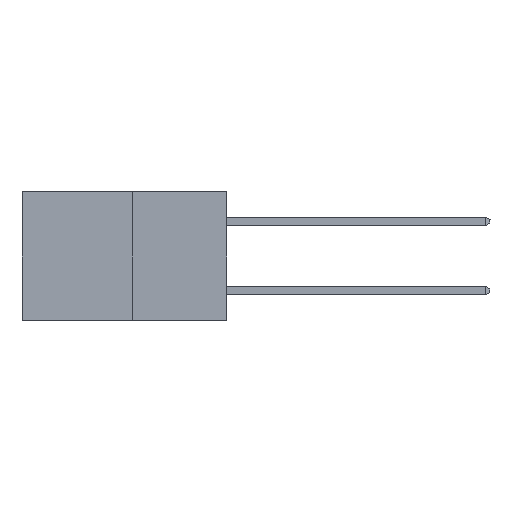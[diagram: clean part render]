
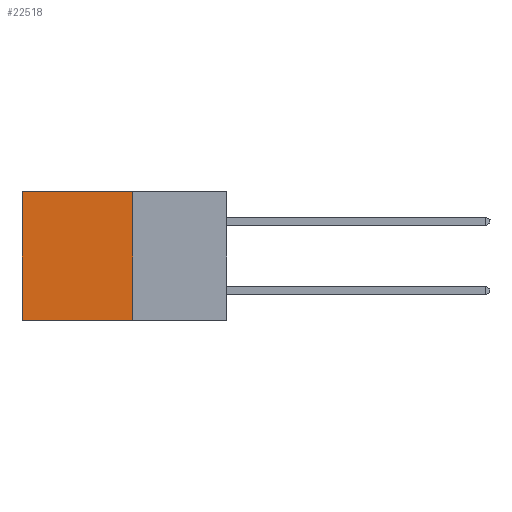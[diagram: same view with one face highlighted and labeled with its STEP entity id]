
A CAD part, left-side view. The second image highlights one B-rep face of the part: STEP entity #22518.
In plain terms, the highlighted planar face has unit normal (-1, 0, 0).
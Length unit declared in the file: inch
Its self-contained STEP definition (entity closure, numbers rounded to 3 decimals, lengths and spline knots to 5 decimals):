
#194 = DIRECTION ( 'NONE',  ( 0., 1., 0. ) ) ;
#245 = CARTESIAN_POINT ( 'NONE',  ( 0.277, 0.27, -0.37 ) ) ;
#1360 = LINE ( 'NONE', #20377, #14068 ) ;
#1440 = VERTEX_POINT ( 'NONE', #5201 ) ;
#2664 = DIRECTION ( 'NONE',  ( 0., 0., -1. ) ) ;
#4241 = ORIENTED_EDGE ( 'NONE', *, *, #16851, .F. ) ;
#5201 = CARTESIAN_POINT ( 'NONE',  ( 0.277, 0.27, 0. ) ) ;
#6169 = VECTOR ( 'NONE', #10595, 39.37008 ) ;
#6457 = EDGE_LOOP ( 'NONE', ( #22980, #4241, #10217, #19124 ) ) ;
#6992 = LINE ( 'NONE', #8060, #6169 ) ;
#8060 = CARTESIAN_POINT ( 'NONE',  ( 0.277, 0.27, 0. ) ) ;
#8202 = VERTEX_POINT ( 'NONE', #9850 ) ;
#9850 = CARTESIAN_POINT ( 'NONE',  ( 0.277, 0.27, -0.37 ) ) ;
#10217 = ORIENTED_EDGE ( 'NONE', *, *, #29340, .F. ) ;
#10595 = DIRECTION ( 'NONE',  ( 0., 1., 0. ) ) ;
#11838 = DIRECTION ( 'NONE',  ( 1., 0., 0. ) ) ;
#14068 = VECTOR ( 'NONE', #2664, 39.37008 ) ;
#14224 = VECTOR ( 'NONE', #194, 39.37008 ) ;
#14652 = LINE ( 'NONE', #245, #27182 ) ;
#15370 = CARTESIAN_POINT ( 'NONE',  ( 0.277, 0.27, -0.37 ) ) ;
#16851 = EDGE_CURVE ( 'NONE', #8202, #30140, #20117, .T. ) ;
#18349 = CARTESIAN_POINT ( 'NONE',  ( 0.277, 0.59, -0.37 ) ) ;
#19122 = EDGE_CURVE ( 'NONE', #31425, #30140, #1360, .T. ) ;
#19124 = ORIENTED_EDGE ( 'NONE', *, *, #25351, .T. ) ;
#20117 = LINE ( 'NONE', #15370, #14224 ) ;
#20247 = CARTESIAN_POINT ( 'NONE',  ( 0.277, 0.59, 0. ) ) ;
#20377 = CARTESIAN_POINT ( 'NONE',  ( 0.277, 0.59, -0.37 ) ) ;
#20483 = DIRECTION ( 'NONE',  ( 0., 0., -1. ) ) ;
#21805 = CARTESIAN_POINT ( 'NONE',  ( 0.277, 0.27, -0.37 ) ) ;
#22518 = ADVANCED_FACE ( 'NONE', ( #25634 ), #26852, .F. ) ;
#22980 = ORIENTED_EDGE ( 'NONE', *, *, #19122, .T. ) ;
#25351 = EDGE_CURVE ( 'NONE', #1440, #31425, #6992, .T. ) ;
#25634 = FACE_OUTER_BOUND ( 'NONE', #6457, .T. ) ;
#26852 = PLANE ( 'NONE',  #28748 ) ;
#27182 = VECTOR ( 'NONE', #20483, 39.37008 ) ;
#28748 = AXIS2_PLACEMENT_3D ( 'NONE', #21805, #11838, #29373 ) ;
#29340 = EDGE_CURVE ( 'NONE', #1440, #8202, #14652, .T. ) ;
#29373 = DIRECTION ( 'NONE',  ( 0., 0., -1. ) ) ;
#30140 = VERTEX_POINT ( 'NONE', #18349 ) ;
#31425 = VERTEX_POINT ( 'NONE', #20247 ) ;
